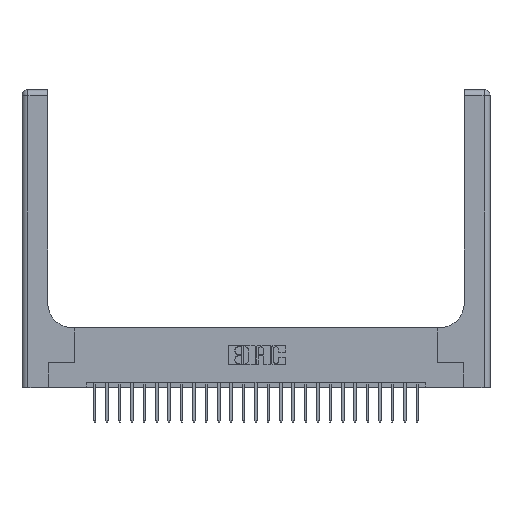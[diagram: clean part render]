
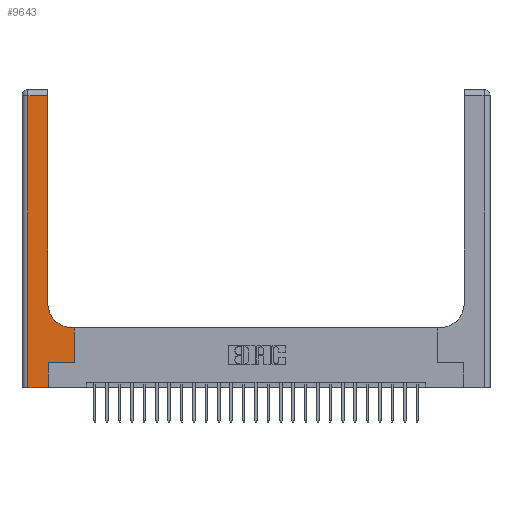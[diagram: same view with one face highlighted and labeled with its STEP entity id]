
A CAD part, top view. The second image highlights one B-rep face of the part: STEP entity #9643.
In plain terms, the highlighted planar face has unit normal (0, 0, 1).
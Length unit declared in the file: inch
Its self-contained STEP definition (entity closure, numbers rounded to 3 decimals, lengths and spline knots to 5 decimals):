
#749 = VECTOR ( 'NONE', #5779, 39.37008 ) ;
#831 = CARTESIAN_POINT ( 'NONE',  ( 0.26, 0.85, 0.37 ) ) ;
#835 = VECTOR ( 'NONE', #20955, 39.37008 ) ;
#851 = ORIENTED_EDGE ( 'NONE', *, *, #17178, .T. ) ;
#875 = DIRECTION ( 'NONE',  ( -1., 0., 0. ) ) ;
#940 = DIRECTION ( 'NONE',  ( 0., -1., 0. ) ) ;
#1352 = VECTOR ( 'NONE', #3342, 39.37008 ) ;
#2515 = VERTEX_POINT ( 'NONE', #831 ) ;
#2682 = DIRECTION ( 'NONE',  ( 0., 1., 0. ) ) ;
#3342 = DIRECTION ( 'NONE',  ( 1., 0., 0. ) ) ;
#3492 = CARTESIAN_POINT ( 'NONE',  ( 0., 3., 0.37 ) ) ;
#3579 = VECTOR ( 'NONE', #15596, 39.37008 ) ;
#4012 = ORIENTED_EDGE ( 'NONE', *, *, #11553, .T. ) ;
#4013 = AXIS2_PLACEMENT_3D ( 'NONE', #18413, #17576, #7974 ) ;
#4790 = VECTOR ( 'NONE', #940, 39.37008 ) ;
#4975 = LINE ( 'NONE', #16512, #20940 ) ;
#5438 = VERTEX_POINT ( 'NONE', #21932 ) ;
#5653 = LINE ( 'NONE', #15536, #749 ) ;
#5779 = DIRECTION ( 'NONE',  ( -1., 0., 0. ) ) ;
#5886 = ORIENTED_EDGE ( 'NONE', *, *, #12556, .T. ) ;
#6138 = ORIENTED_EDGE ( 'NONE', *, *, #20120, .T. ) ;
#6193 = LINE ( 'NONE', #18359, #4790 ) ;
#6755 = CARTESIAN_POINT ( 'NONE',  ( 0., 2.94, 0.37 ) ) ;
#7212 = DIRECTION ( 'NONE',  ( 0., 0., -1. ) ) ;
#7974 = DIRECTION ( 'NONE',  ( 1., 0., 0. ) ) ;
#8897 = VECTOR ( 'NONE', #22614, 39.37008 ) ;
#9026 = CARTESIAN_POINT ( 'NONE',  ( 0.06, 2.94, 0.37 ) ) ;
#9643 = ADVANCED_FACE ( 'NONE', ( #13497 ), #19115, .F. ) ;
#11241 = CARTESIAN_POINT ( 'NONE',  ( 0.265, 0., 0.37 ) ) ;
#11553 = EDGE_CURVE ( 'NONE', #13925, #12062, #23765, .T. ) ;
#11622 = CARTESIAN_POINT ( 'NONE',  ( 0.265, 0.25, 0.37 ) ) ;
#11790 = CIRCLE ( 'NONE', #4013, 0.25 ) ;
#12062 = VERTEX_POINT ( 'NONE', #20477 ) ;
#12556 = EDGE_CURVE ( 'NONE', #17070, #19216, #14710, .T. ) ;
#12768 = LINE ( 'NONE', #11241, #835 ) ;
#13108 = DIRECTION ( 'NONE',  ( -1., 0., 0. ) ) ;
#13250 = EDGE_CURVE ( 'NONE', #19216, #5438, #6193, .T. ) ;
#13497 = FACE_OUTER_BOUND ( 'NONE', #15893, .T. ) ;
#13708 = CARTESIAN_POINT ( 'NONE',  ( 0.528, 0.6, 0.37 ) ) ;
#13925 = VERTEX_POINT ( 'NONE', #23903 ) ;
#14182 = ORIENTED_EDGE ( 'NONE', *, *, #24875, .T. ) ;
#14710 = LINE ( 'NONE', #6755, #21969 ) ;
#14748 = CARTESIAN_POINT ( 'NONE',  ( 0., 0., 0.37 ) ) ;
#14868 = EDGE_CURVE ( 'NONE', #2515, #17070, #16494, .T. ) ;
#15536 = CARTESIAN_POINT ( 'NONE',  ( 0.26, 0.6, 0.37 ) ) ;
#15557 = ORIENTED_EDGE ( 'NONE', *, *, #23917, .T. ) ;
#15596 = DIRECTION ( 'NONE',  ( 1., 0., 0. ) ) ;
#15893 = EDGE_LOOP ( 'NONE', ( #21262, #5886, #22943, #14182, #6138, #4012, #15557, #851, #20229 ) ) ;
#15896 = VERTEX_POINT ( 'NONE', #13708 ) ;
#16494 = LINE ( 'NONE', #16998, #8897 ) ;
#16512 = CARTESIAN_POINT ( 'NONE',  ( 0.528, 0.25, 0.37 ) ) ;
#16617 = CARTESIAN_POINT ( 'NONE',  ( 0.265, 0., 0.37 ) ) ;
#16927 = LINE ( 'NONE', #14748, #1352 ) ;
#16998 = CARTESIAN_POINT ( 'NONE',  ( 0.26, 3., 0.37 ) ) ;
#17070 = VERTEX_POINT ( 'NONE', #24106 ) ;
#17178 = EDGE_CURVE ( 'NONE', #15896, #18005, #5653, .T. ) ;
#17287 = EDGE_CURVE ( 'NONE', #18005, #2515, #11790, .T. ) ;
#17576 = DIRECTION ( 'NONE',  ( 0., 0., -1. ) ) ;
#18005 = VERTEX_POINT ( 'NONE', #23094 ) ;
#18359 = CARTESIAN_POINT ( 'NONE',  ( 0.06, 3., 0.37 ) ) ;
#18413 = CARTESIAN_POINT ( 'NONE',  ( 0.51, 0.85, 0.37 ) ) ;
#18720 = VERTEX_POINT ( 'NONE', #16617 ) ;
#19115 = PLANE ( 'NONE',  #23638 ) ;
#19216 = VERTEX_POINT ( 'NONE', #9026 ) ;
#20120 = EDGE_CURVE ( 'NONE', #18720, #13925, #12768, .T. ) ;
#20229 = ORIENTED_EDGE ( 'NONE', *, *, #17287, .T. ) ;
#20477 = CARTESIAN_POINT ( 'NONE',  ( 0.528, 0.25, 0.37 ) ) ;
#20940 = VECTOR ( 'NONE', #2682, 39.37008 ) ;
#20955 = DIRECTION ( 'NONE',  ( 0., 1., 0. ) ) ;
#21262 = ORIENTED_EDGE ( 'NONE', *, *, #14868, .T. ) ;
#21932 = CARTESIAN_POINT ( 'NONE',  ( 0.06, 0., 0.37 ) ) ;
#21969 = VECTOR ( 'NONE', #875, 39.37008 ) ;
#22614 = DIRECTION ( 'NONE',  ( 0., 1., 0. ) ) ;
#22943 = ORIENTED_EDGE ( 'NONE', *, *, #13250, .T. ) ;
#23094 = CARTESIAN_POINT ( 'NONE',  ( 0.51, 0.6, 0.37 ) ) ;
#23638 = AXIS2_PLACEMENT_3D ( 'NONE', #3492, #7212, #13108 ) ;
#23765 = LINE ( 'NONE', #11622, #3579 ) ;
#23903 = CARTESIAN_POINT ( 'NONE',  ( 0.265, 0.25, 0.37 ) ) ;
#23917 = EDGE_CURVE ( 'NONE', #12062, #15896, #4975, .T. ) ;
#24106 = CARTESIAN_POINT ( 'NONE',  ( 0.26, 2.94, 0.37 ) ) ;
#24875 = EDGE_CURVE ( 'NONE', #5438, #18720, #16927, .T. ) ;
